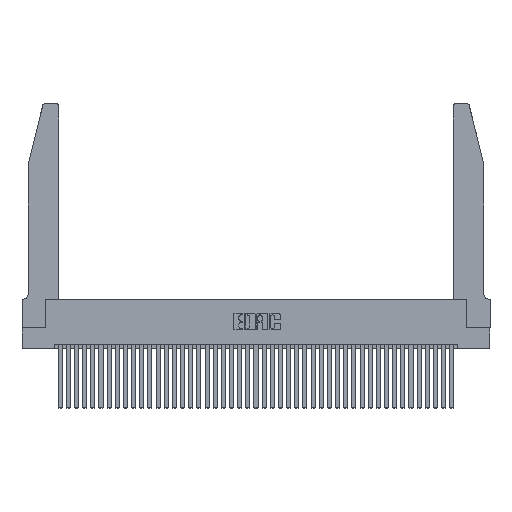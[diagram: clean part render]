
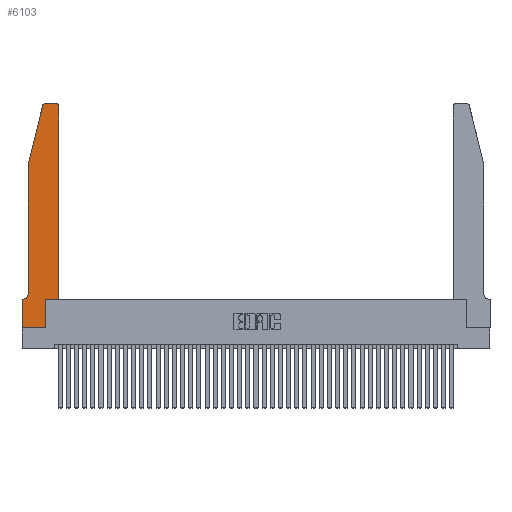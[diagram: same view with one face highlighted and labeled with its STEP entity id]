
A CAD part, top view. The second image highlights one B-rep face of the part: STEP entity #6103.
In plain terms, the highlighted planar face has unit normal (0, 0, 1).
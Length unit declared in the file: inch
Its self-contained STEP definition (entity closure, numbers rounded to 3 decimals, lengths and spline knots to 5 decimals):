
#388 = EDGE_CURVE ( 'NONE', #12533, #7294, #32919, .T. ) ;
#828 = DIRECTION ( 'NONE',  ( 0., 1., 0. ) ) ;
#862 = ORIENTED_EDGE ( 'NONE', *, *, #388, .T. ) ;
#1127 = CARTESIAN_POINT ( 'NONE',  ( 0., 0., 0.37 ) ) ;
#1629 = EDGE_CURVE ( 'NONE', #26243, #38069, #30288, .T. ) ;
#2273 = DIRECTION ( 'NONE',  ( -1., 0., 0. ) ) ;
#2522 = ORIENTED_EDGE ( 'NONE', *, *, #35465, .T. ) ;
#2629 = AXIS2_PLACEMENT_3D ( 'NONE', #31685, #30599, #30482 ) ;
#2731 = LINE ( 'NONE', #13041, #28701 ) ;
#2914 = EDGE_CURVE ( 'NONE', #13759, #10769, #32679, .T. ) ;
#3097 = LINE ( 'NONE', #1127, #20454 ) ;
#3505 = CARTESIAN_POINT ( 'NONE',  ( 0.4505, 2.72, 0.37 ) ) ;
#3765 = AXIS2_PLACEMENT_3D ( 'NONE', #7891, #30622, #11158 ) ;
#4252 = EDGE_CURVE ( 'NONE', #13654, #26243, #9712, .T. ) ;
#4577 = CARTESIAN_POINT ( 'NONE',  ( 0.4505, 0.35, 0.37 ) ) ;
#5502 = ORIENTED_EDGE ( 'NONE', *, *, #1629, .T. ) ;
#6103 = ADVANCED_FACE ( 'NONE', ( #27758 ), #42045, .T. ) ;
#6563 = DIRECTION ( 'NONE',  ( 1., 0., 0. ) ) ;
#7294 = VERTEX_POINT ( 'NONE', #8910 ) ;
#7571 = DIRECTION ( 'NONE',  ( -0.239, -0.971, 0. ) ) ;
#7891 = CARTESIAN_POINT ( 'NONE',  ( 0.0055, 0.42, 0.37 ) ) ;
#8516 = DIRECTION ( 'NONE',  ( 0., 1., 0. ) ) ;
#8568 = CIRCLE ( 'NONE', #18854, 0.03 ) ;
#8910 = CARTESIAN_POINT ( 'NONE',  ( 0.25487, 2.72718, 0.37 ) ) ;
#9712 = LINE ( 'NONE', #38497, #34572 ) ;
#10769 = VERTEX_POINT ( 'NONE', #38376 ) ;
#10776 = VERTEX_POINT ( 'NONE', #12439 ) ;
#11158 = DIRECTION ( 'NONE',  ( -1., 0., 0. ) ) ;
#12439 = CARTESIAN_POINT ( 'NONE',  ( 0.4205, 2.75, 0.37 ) ) ;
#12533 = VERTEX_POINT ( 'NONE', #31762 ) ;
#13023 = EDGE_LOOP ( 'NONE', ( #15274, #862, #36003, #41540, #5502, #33078, #15854, #2522, #19653, #21693, #24757, #16672 ) ) ;
#13041 = CARTESIAN_POINT ( 'NONE',  ( 0.2605, 2.75, 0.37 ) ) ;
#13654 = VERTEX_POINT ( 'NONE', #34774 ) ;
#13759 = VERTEX_POINT ( 'NONE', #15782 ) ;
#14913 = AXIS2_PLACEMENT_3D ( 'NONE', #16260, #26073, #6563 ) ;
#15274 = ORIENTED_EDGE ( 'NONE', *, *, #17975, .T. ) ;
#15782 = CARTESIAN_POINT ( 'NONE',  ( 0.2865, 0., 0.37 ) ) ;
#15848 = DIRECTION ( 'NONE',  ( 0., 0., 1. ) ) ;
#15854 = ORIENTED_EDGE ( 'NONE', *, *, #23608, .T. ) ;
#16260 = CARTESIAN_POINT ( 'NONE',  ( 0., 0.35, 0.37 ) ) ;
#16308 = DIRECTION ( 'NONE',  ( 1., 0., 0. ) ) ;
#16672 = ORIENTED_EDGE ( 'NONE', *, *, #27301, .T. ) ;
#16718 = CARTESIAN_POINT ( 'NONE',  ( 0.0055, 0.35, 0.37 ) ) ;
#17975 = EDGE_CURVE ( 'NONE', #10776, #12533, #2731, .T. ) ;
#17987 = EDGE_CURVE ( 'NONE', #10769, #23914, #19084, .T. ) ;
#18854 = AXIS2_PLACEMENT_3D ( 'NONE', #35264, #15848, #38513 ) ;
#19084 = LINE ( 'NONE', #22846, #35298 ) ;
#19104 = DIRECTION ( 'NONE',  ( 0., -1., 0. ) ) ;
#19650 = LINE ( 'NONE', #23658, #37852 ) ;
#19653 = ORIENTED_EDGE ( 'NONE', *, *, #2914, .T. ) ;
#20454 = VECTOR ( 'NONE', #23953, 39.37008 ) ;
#21547 = VERTEX_POINT ( 'NONE', #25583 ) ;
#21693 = ORIENTED_EDGE ( 'NONE', *, *, #17987, .T. ) ;
#22846 = CARTESIAN_POINT ( 'NONE',  ( 0.4505, 0.35, 0.37 ) ) ;
#23608 = EDGE_CURVE ( 'NONE', #21547, #31498, #24320, .T. ) ;
#23658 = CARTESIAN_POINT ( 'NONE',  ( 0.4505, 0.35, 0.37 ) ) ;
#23794 = CARTESIAN_POINT ( 'NONE',  ( 0.0755, 2., 0.37 ) ) ;
#23914 = VERTEX_POINT ( 'NONE', #4577 ) ;
#23953 = DIRECTION ( 'NONE',  ( 1., 0., 0. ) ) ;
#24320 = LINE ( 'NONE', #35344, #39524 ) ;
#24757 = ORIENTED_EDGE ( 'NONE', *, *, #41613, .T. ) ;
#25583 = CARTESIAN_POINT ( 'NONE',  ( 0., 0.35, 0.37 ) ) ;
#26073 = DIRECTION ( 'NONE',  ( 0., 0., 1. ) ) ;
#26243 = VERTEX_POINT ( 'NONE', #29993 ) ;
#26585 = CARTESIAN_POINT ( 'NONE',  ( 0., 0., 0.37 ) ) ;
#27301 = EDGE_CURVE ( 'NONE', #31423, #10776, #8568, .T. ) ;
#27758 = FACE_OUTER_BOUND ( 'NONE', #13023, .T. ) ;
#28335 = CARTESIAN_POINT ( 'NONE',  ( 0.0755, 0.35, 0.37 ) ) ;
#28701 = VECTOR ( 'NONE', #38986, 39.37008 ) ;
#29993 = CARTESIAN_POINT ( 'NONE',  ( 0.0755, 0.42, 0.37 ) ) ;
#30288 = CIRCLE ( 'NONE', #3765, 0.07 ) ;
#30482 = DIRECTION ( 'NONE',  ( 1., 0., 0. ) ) ;
#30599 = DIRECTION ( 'NONE',  ( 0., 0., 1. ) ) ;
#30622 = DIRECTION ( 'NONE',  ( 0., 0., -1. ) ) ;
#31423 = VERTEX_POINT ( 'NONE', #3505 ) ;
#31498 = VERTEX_POINT ( 'NONE', #26585 ) ;
#31685 = CARTESIAN_POINT ( 'NONE',  ( 0.284, 2.72, 0.37 ) ) ;
#31762 = CARTESIAN_POINT ( 'NONE',  ( 0.284, 2.75, 0.37 ) ) ;
#32406 = EDGE_CURVE ( 'NONE', #38069, #21547, #32892, .T. ) ;
#32679 = LINE ( 'NONE', #40844, #40263 ) ;
#32838 = EDGE_CURVE ( 'NONE', #7294, #13654, #33836, .T. ) ;
#32892 = LINE ( 'NONE', #28335, #39464 ) ;
#32919 = CIRCLE ( 'NONE', #2629, 0.03 ) ;
#33078 = ORIENTED_EDGE ( 'NONE', *, *, #32406, .T. ) ;
#33836 = LINE ( 'NONE', #23794, #40424 ) ;
#34572 = VECTOR ( 'NONE', #19104, 39.37008 ) ;
#34774 = CARTESIAN_POINT ( 'NONE',  ( 0.0755, 2., 0.37 ) ) ;
#35264 = CARTESIAN_POINT ( 'NONE',  ( 0.4205, 2.72, 0.37 ) ) ;
#35298 = VECTOR ( 'NONE', #16308, 39.37008 ) ;
#35344 = CARTESIAN_POINT ( 'NONE',  ( 0., 0., 0.37 ) ) ;
#35465 = EDGE_CURVE ( 'NONE', #31498, #13759, #3097, .T. ) ;
#35622 = DIRECTION ( 'NONE',  ( 0., -1., 0. ) ) ;
#36003 = ORIENTED_EDGE ( 'NONE', *, *, #32838, .T. ) ;
#37852 = VECTOR ( 'NONE', #828, 39.37008 ) ;
#38069 = VERTEX_POINT ( 'NONE', #16718 ) ;
#38376 = CARTESIAN_POINT ( 'NONE',  ( 0.2865, 0.35, 0.37 ) ) ;
#38497 = CARTESIAN_POINT ( 'NONE',  ( 0.0755, 2., 0.37 ) ) ;
#38513 = DIRECTION ( 'NONE',  ( 1., 0., 0. ) ) ;
#38986 = DIRECTION ( 'NONE',  ( -1., 0., 0. ) ) ;
#39464 = VECTOR ( 'NONE', #2273, 39.37008 ) ;
#39524 = VECTOR ( 'NONE', #35622, 39.37008 ) ;
#40263 = VECTOR ( 'NONE', #8516, 39.37008 ) ;
#40424 = VECTOR ( 'NONE', #7571, 39.37008 ) ;
#40844 = CARTESIAN_POINT ( 'NONE',  ( 0.2865, 0.35, 0.37 ) ) ;
#41540 = ORIENTED_EDGE ( 'NONE', *, *, #4252, .T. ) ;
#41613 = EDGE_CURVE ( 'NONE', #23914, #31423, #19650, .T. ) ;
#42045 = PLANE ( 'NONE',  #14913 ) ;
